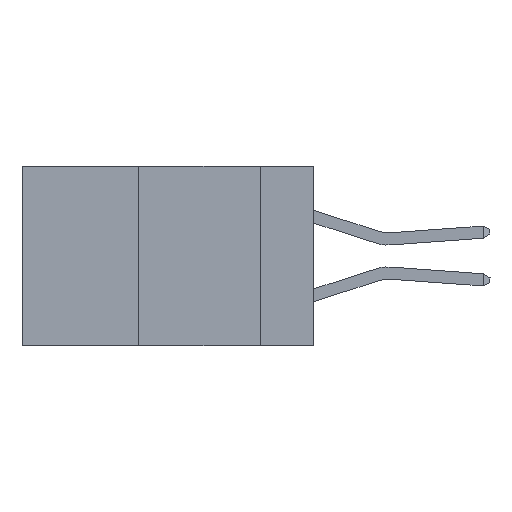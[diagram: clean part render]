
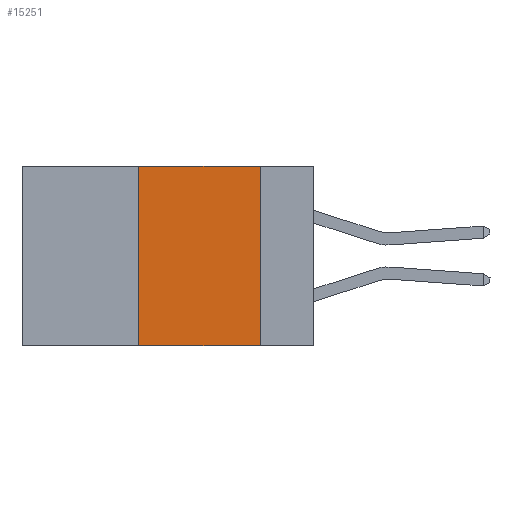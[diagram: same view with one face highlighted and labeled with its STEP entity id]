
A CAD part, left-side view. The second image highlights one B-rep face of the part: STEP entity #15251.
In plain terms, the highlighted planar face has unit normal (-1, 0, 0).
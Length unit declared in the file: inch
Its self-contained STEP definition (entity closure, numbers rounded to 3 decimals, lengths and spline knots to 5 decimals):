
#69 = VERTEX_POINT ( 'NONE', #20825 ) ;
#283 = DIRECTION ( 'NONE',  ( 0., 0., 1. ) ) ;
#348 = DIRECTION ( 'NONE',  ( 1., 0., 0. ) ) ;
#1215 = CARTESIAN_POINT ( 'NONE',  ( 0., 0.36, -0.37 ) ) ;
#1480 = LINE ( 'NONE', #16116, #10354 ) ;
#1562 = ORIENTED_EDGE ( 'NONE', *, *, #9340, .F. ) ;
#1793 = VERTEX_POINT ( 'NONE', #1215 ) ;
#2466 = EDGE_LOOP ( 'NONE', ( #1562, #21077, #12179, #7544 ) ) ;
#2582 = LINE ( 'NONE', #21171, #15062 ) ;
#3017 = CARTESIAN_POINT ( 'NONE',  ( 0., 0.11, 0. ) ) ;
#3878 = PLANE ( 'NONE',  #20713 ) ;
#5299 = LINE ( 'NONE', #3017, #9415 ) ;
#7544 = ORIENTED_EDGE ( 'NONE', *, *, #15220, .T. ) ;
#9340 = EDGE_CURVE ( 'NONE', #69, #11982, #5299, .T. ) ;
#9415 = VECTOR ( 'NONE', #15379, 39.37008 ) ;
#10335 = EDGE_CURVE ( 'NONE', #1793, #10659, #11412, .T. ) ;
#10354 = VECTOR ( 'NONE', #19606, 39.37008 ) ;
#10659 = VERTEX_POINT ( 'NONE', #11746 ) ;
#10899 = CARTESIAN_POINT ( 'NONE',  ( 0., 0.36, 0. ) ) ;
#10967 = CARTESIAN_POINT ( 'NONE',  ( 0., 0.6, 0. ) ) ;
#11412 = LINE ( 'NONE', #10899, #20660 ) ;
#11746 = CARTESIAN_POINT ( 'NONE',  ( 0., 0.36, 0. ) ) ;
#11982 = VERTEX_POINT ( 'NONE', #20439 ) ;
#12179 = ORIENTED_EDGE ( 'NONE', *, *, #10335, .F. ) ;
#12575 = DIRECTION ( 'NONE',  ( 0., -1., 0. ) ) ;
#12781 = DIRECTION ( 'NONE',  ( 0., 0., -1. ) ) ;
#14544 = FACE_OUTER_BOUND ( 'NONE', #2466, .T. ) ;
#15062 = VECTOR ( 'NONE', #12575, 39.37008 ) ;
#15220 = EDGE_CURVE ( 'NONE', #1793, #11982, #1480, .T. ) ;
#15251 = ADVANCED_FACE ( 'NONE', ( #14544 ), #3878, .F. ) ;
#15379 = DIRECTION ( 'NONE',  ( 0., 0., -1. ) ) ;
#15901 = EDGE_CURVE ( 'NONE', #10659, #69, #2582, .T. ) ;
#16116 = CARTESIAN_POINT ( 'NONE',  ( 0., 0.6, -0.37 ) ) ;
#19606 = DIRECTION ( 'NONE',  ( 0., -1., 0. ) ) ;
#20439 = CARTESIAN_POINT ( 'NONE',  ( 0., 0.11, -0.37 ) ) ;
#20660 = VECTOR ( 'NONE', #283, 39.37008 ) ;
#20713 = AXIS2_PLACEMENT_3D ( 'NONE', #10967, #348, #12781 ) ;
#20825 = CARTESIAN_POINT ( 'NONE',  ( 0., 0.11, 0. ) ) ;
#21077 = ORIENTED_EDGE ( 'NONE', *, *, #15901, .F. ) ;
#21171 = CARTESIAN_POINT ( 'NONE',  ( 0., 0.6, 0. ) ) ;
